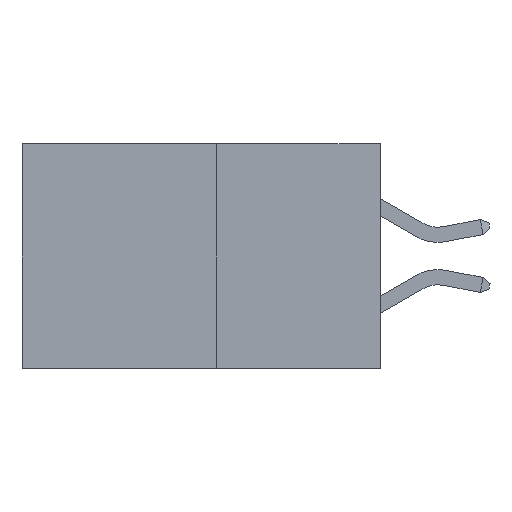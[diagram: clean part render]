
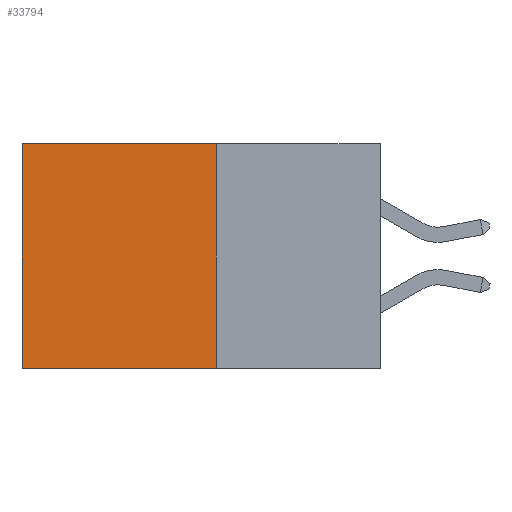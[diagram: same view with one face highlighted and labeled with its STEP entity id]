
A CAD part, left-side view. The second image highlights one B-rep face of the part: STEP entity #33794.
In plain terms, the highlighted planar face has unit normal (-1, 0, 0).
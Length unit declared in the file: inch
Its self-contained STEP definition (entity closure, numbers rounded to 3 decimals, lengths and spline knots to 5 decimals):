
#373 = VECTOR ( 'NONE', #23870, 39.37008 ) ;
#3991 = CARTESIAN_POINT ( 'NONE',  ( 0.277, 0.27, -0.37 ) ) ;
#4385 = EDGE_CURVE ( 'NONE', #5413, #33704, #8077, .T. ) ;
#5413 = VERTEX_POINT ( 'NONE', #27081 ) ;
#6050 = CARTESIAN_POINT ( 'NONE',  ( 0.277, 0.27, -0.37 ) ) ;
#6168 = VECTOR ( 'NONE', #17470, 39.37008 ) ;
#6767 = ORIENTED_EDGE ( 'NONE', *, *, #14692, .F. ) ;
#8077 = LINE ( 'NONE', #35880, #29692 ) ;
#10479 = VERTEX_POINT ( 'NONE', #11989 ) ;
#11989 = CARTESIAN_POINT ( 'NONE',  ( 0.277, 0.27, -0.37 ) ) ;
#14638 = LINE ( 'NONE', #6050, #6168 ) ;
#14673 = LINE ( 'NONE', #3991, #373 ) ;
#14692 = EDGE_CURVE ( 'NONE', #5413, #10479, #14673, .T. ) ;
#14776 = ORIENTED_EDGE ( 'NONE', *, *, #4385, .T. ) ;
#15576 = AXIS2_PLACEMENT_3D ( 'NONE', #24135, #32567, #15739 ) ;
#15739 = DIRECTION ( 'NONE',  ( 0., 0., -1. ) ) ;
#16958 = VECTOR ( 'NONE', #35731, 39.37008 ) ;
#17172 = FACE_OUTER_BOUND ( 'NONE', #30740, .T. ) ;
#17470 = DIRECTION ( 'NONE',  ( 0., 1., 0. ) ) ;
#17845 = LINE ( 'NONE', #30141, #16958 ) ;
#18444 = PLANE ( 'NONE',  #15576 ) ;
#22851 = CARTESIAN_POINT ( 'NONE',  ( 0.277, 0.59, -0.37 ) ) ;
#23870 = DIRECTION ( 'NONE',  ( 0., 0., -1. ) ) ;
#24135 = CARTESIAN_POINT ( 'NONE',  ( 0.277, 0.27, -0.37 ) ) ;
#27081 = CARTESIAN_POINT ( 'NONE',  ( 0.277, 0.27, 0. ) ) ;
#29386 = CARTESIAN_POINT ( 'NONE',  ( 0.277, 0.59, 0. ) ) ;
#29692 = VECTOR ( 'NONE', #33340, 39.37008 ) ;
#30141 = CARTESIAN_POINT ( 'NONE',  ( 0.277, 0.59, -0.37 ) ) ;
#30159 = ORIENTED_EDGE ( 'NONE', *, *, #31859, .F. ) ;
#30181 = EDGE_CURVE ( 'NONE', #33704, #32477, #17845, .T. ) ;
#30409 = ORIENTED_EDGE ( 'NONE', *, *, #30181, .T. ) ;
#30740 = EDGE_LOOP ( 'NONE', ( #30409, #30159, #6767, #14776 ) ) ;
#31859 = EDGE_CURVE ( 'NONE', #10479, #32477, #14638, .T. ) ;
#32477 = VERTEX_POINT ( 'NONE', #22851 ) ;
#32567 = DIRECTION ( 'NONE',  ( 1., 0., 0. ) ) ;
#33340 = DIRECTION ( 'NONE',  ( 0., 1., 0. ) ) ;
#33704 = VERTEX_POINT ( 'NONE', #29386 ) ;
#33794 = ADVANCED_FACE ( 'NONE', ( #17172 ), #18444, .F. ) ;
#35731 = DIRECTION ( 'NONE',  ( 0., 0., -1. ) ) ;
#35880 = CARTESIAN_POINT ( 'NONE',  ( 0.277, 0.27, 0. ) ) ;
